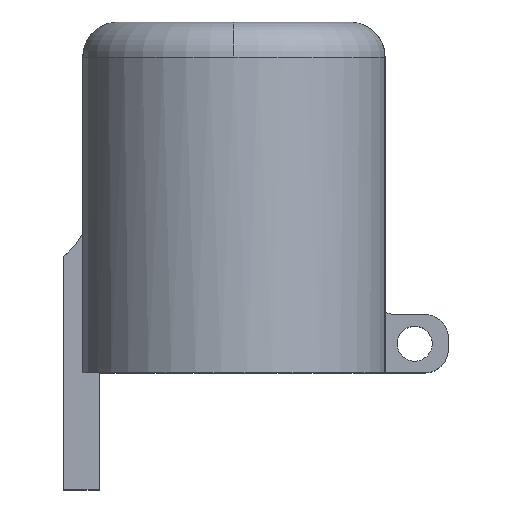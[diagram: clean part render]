
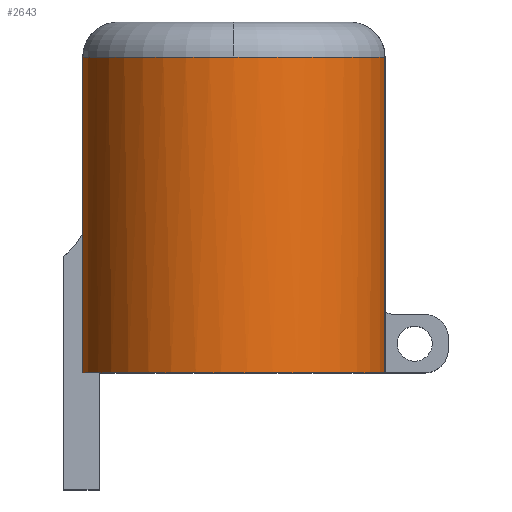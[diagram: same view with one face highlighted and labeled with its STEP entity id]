
A CAD part, top view. The second image highlights one B-rep face of the part: STEP entity #2643.
In plain terms, the highlighted cylindrical face has radius 33.02 mm (diameter 66.04 mm), a partial arc.
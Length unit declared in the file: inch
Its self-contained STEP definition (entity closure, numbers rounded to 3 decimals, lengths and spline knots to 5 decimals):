
#24 = CARTESIAN_POINT ( 'NONE',  ( 0., 2.7, 0. ) ) ;
#53 = VERTEX_POINT ( 'NONE', #873 ) ;
#157 = ORIENTED_EDGE ( 'NONE', *, *, #3078, .T. ) ;
#207 = DIRECTION ( 'NONE',  ( 0., -1., 0. ) ) ;
#273 = CIRCLE ( 'NONE', #2889, 1.3 ) ;
#325 = LINE ( 'NONE', #655, #708 ) ;
#368 = FACE_OUTER_BOUND ( 'NONE', #506, .T. ) ;
#416 = CIRCLE ( 'NONE', #3277, 1.3 ) ;
#495 = VECTOR ( 'NONE', #1953, 39.37008 ) ;
#506 = EDGE_LOOP ( 'NONE', ( #638, #908, #1695, #2919, #157 ) ) ;
#638 = ORIENTED_EDGE ( 'NONE', *, *, #1383, .T. ) ;
#655 = CARTESIAN_POINT ( 'NONE',  ( -1.29068, 3., 0.15535 ) ) ;
#708 = VECTOR ( 'NONE', #2054, 39.37008 ) ;
#873 = CARTESIAN_POINT ( 'NONE',  ( 1.29115, 0., 0.15144 ) ) ;
#908 = ORIENTED_EDGE ( 'NONE', *, *, #1265, .T. ) ;
#1107 = CARTESIAN_POINT ( 'NONE',  ( 0., 0., 0. ) ) ;
#1265 = EDGE_CURVE ( 'NONE', #2894, #2811, #416, .T. ) ;
#1352 = DIRECTION ( 'NONE',  ( 0., 0., 1. ) ) ;
#1383 = EDGE_CURVE ( 'NONE', #53, #2894, #1988, .T. ) ;
#1539 = CARTESIAN_POINT ( 'NONE',  ( 0., 3., 0. ) ) ;
#1582 = EDGE_CURVE ( 'NONE', #2333, #2409, #325, .T. ) ;
#1606 = CARTESIAN_POINT ( 'NONE',  ( 1.29115, 2.7, 0.15144 ) ) ;
#1629 = EDGE_CURVE ( 'NONE', #2811, #2333, #3236, .T. ) ;
#1695 = ORIENTED_EDGE ( 'NONE', *, *, #1629, .T. ) ;
#1754 = AXIS2_PLACEMENT_3D ( 'NONE', #1539, #207, #2336 ) ;
#1856 = CARTESIAN_POINT ( 'NONE',  ( 0., 2.7, 1.3 ) ) ;
#1871 = CARTESIAN_POINT ( 'NONE',  ( -1.29068, 0., 0.15535 ) ) ;
#1910 = CARTESIAN_POINT ( 'NONE',  ( -1.29068, 2.7, 0.15535 ) ) ;
#1953 = DIRECTION ( 'NONE',  ( 0., 1., 0. ) ) ;
#1988 = LINE ( 'NONE', #3056, #495 ) ;
#2054 = DIRECTION ( 'NONE',  ( 0., -1., 0. ) ) ;
#2088 = DIRECTION ( 'NONE',  ( 0., -1., 0. ) ) ;
#2181 = DIRECTION ( 'NONE',  ( 0., 1., 0. ) ) ;
#2308 = CARTESIAN_POINT ( 'NONE',  ( 0., 2.7, 0. ) ) ;
#2333 = VERTEX_POINT ( 'NONE', #1910 ) ;
#2336 = DIRECTION ( 'NONE',  ( 0., 0., -1. ) ) ;
#2409 = VERTEX_POINT ( 'NONE', #1871 ) ;
#2643 = ADVANCED_FACE ( 'NONE', ( #368 ), #2984, .T. ) ;
#2748 = AXIS2_PLACEMENT_3D ( 'NONE', #2308, #2088, #3485 ) ;
#2811 = VERTEX_POINT ( 'NONE', #1856 ) ;
#2889 = AXIS2_PLACEMENT_3D ( 'NONE', #1107, #2181, #3431 ) ;
#2894 = VERTEX_POINT ( 'NONE', #1606 ) ;
#2919 = ORIENTED_EDGE ( 'NONE', *, *, #1582, .T. ) ;
#2957 = DIRECTION ( 'NONE',  ( 0., -1., 0. ) ) ;
#2984 = CYLINDRICAL_SURFACE ( 'NONE', #1754, 1.3 ) ;
#3056 = CARTESIAN_POINT ( 'NONE',  ( 1.29115, 3., 0.15144 ) ) ;
#3078 = EDGE_CURVE ( 'NONE', #2409, #53, #273, .T. ) ;
#3236 = CIRCLE ( 'NONE', #2748, 1.3 ) ;
#3277 = AXIS2_PLACEMENT_3D ( 'NONE', #24, #2957, #1352 ) ;
#3431 = DIRECTION ( 'NONE',  ( 0., 0., 1. ) ) ;
#3485 = DIRECTION ( 'NONE',  ( 0., 0., 1. ) ) ;
